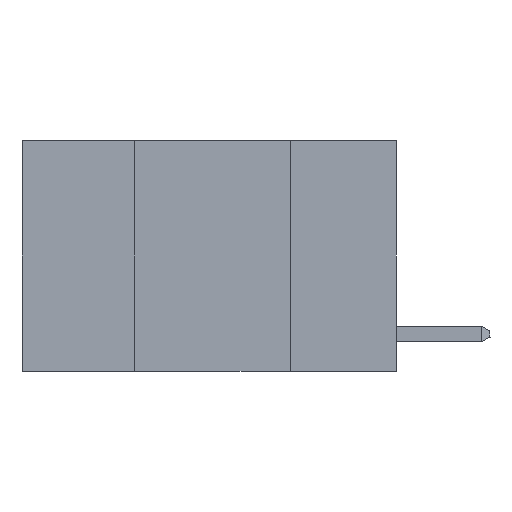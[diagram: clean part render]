
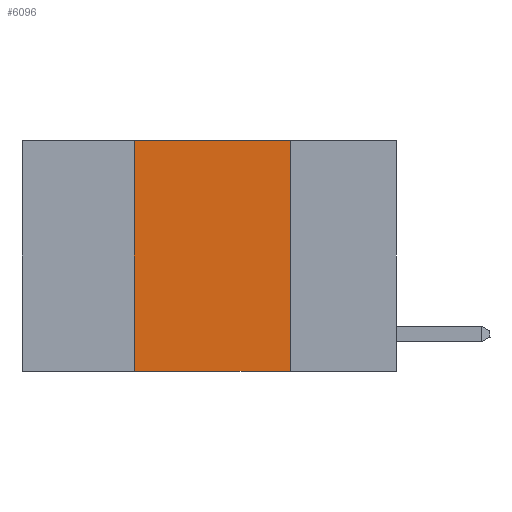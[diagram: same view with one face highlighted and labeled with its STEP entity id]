
A CAD part, left-side view. The second image highlights one B-rep face of the part: STEP entity #6096.
In plain terms, the highlighted planar face has unit normal (-1, 0, 0).
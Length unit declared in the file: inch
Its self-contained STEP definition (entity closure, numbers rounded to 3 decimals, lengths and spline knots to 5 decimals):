
#703 = VERTEX_POINT ( 'NONE', #11160 ) ;
#1280 = LINE ( 'NONE', #9103, #7799 ) ;
#1834 = EDGE_CURVE ( 'NONE', #3812, #3307, #11126, .T. ) ;
#1981 = VECTOR ( 'NONE', #5624, 39.37008 ) ;
#2698 = ORIENTED_EDGE ( 'NONE', *, *, #6928, .T. ) ;
#3307 = VERTEX_POINT ( 'NONE', #4515 ) ;
#3812 = VERTEX_POINT ( 'NONE', #14347 ) ;
#3843 = ORIENTED_EDGE ( 'NONE', *, *, #1834, .F. ) ;
#3962 = FACE_OUTER_BOUND ( 'NONE', #10571, .T. ) ;
#4505 = CARTESIAN_POINT ( 'NONE',  ( 0., 0.42, 0. ) ) ;
#4515 = CARTESIAN_POINT ( 'NONE',  ( 0., 0.17, 0. ) ) ;
#5047 = DIRECTION ( 'NONE',  ( 0., 0., -1. ) ) ;
#5151 = DIRECTION ( 'NONE',  ( 1., 0., 0. ) ) ;
#5517 = CARTESIAN_POINT ( 'NONE',  ( 0., 0.6, 0. ) ) ;
#5624 = DIRECTION ( 'NONE',  ( 0., 0., 1. ) ) ;
#6096 = ADVANCED_FACE ( 'NONE', ( #3962 ), #11874, .F. ) ;
#6123 = CARTESIAN_POINT ( 'NONE',  ( 0., 0.42, -0.37 ) ) ;
#6208 = CARTESIAN_POINT ( 'NONE',  ( 0., 0.6, 0. ) ) ;
#6257 = CARTESIAN_POINT ( 'NONE',  ( 0., 0.17, 0. ) ) ;
#6723 = DIRECTION ( 'NONE',  ( 0., -1., 0. ) ) ;
#6928 = EDGE_CURVE ( 'NONE', #13178, #703, #1280, .T. ) ;
#7799 = VECTOR ( 'NONE', #6723, 39.37008 ) ;
#8449 = VECTOR ( 'NONE', #5047, 39.37008 ) ;
#8719 = LINE ( 'NONE', #6257, #8449 ) ;
#9103 = CARTESIAN_POINT ( 'NONE',  ( 0., 0.6, -0.37 ) ) ;
#10084 = DIRECTION ( 'NONE',  ( 0., -1., 0. ) ) ;
#10571 = EDGE_LOOP ( 'NONE', ( #14606, #3843, #12795, #2698 ) ) ;
#11126 = LINE ( 'NONE', #5517, #13685 ) ;
#11160 = CARTESIAN_POINT ( 'NONE',  ( 0., 0.17, -0.37 ) ) ;
#11522 = EDGE_CURVE ( 'NONE', #13178, #3812, #13768, .T. ) ;
#11874 = PLANE ( 'NONE',  #13803 ) ;
#12795 = ORIENTED_EDGE ( 'NONE', *, *, #11522, .F. ) ;
#13178 = VERTEX_POINT ( 'NONE', #6123 ) ;
#13685 = VECTOR ( 'NONE', #10084, 39.37008 ) ;
#13768 = LINE ( 'NONE', #4505, #1981 ) ;
#13803 = AXIS2_PLACEMENT_3D ( 'NONE', #6208, #5151, #13913 ) ;
#13913 = DIRECTION ( 'NONE',  ( 0., 0., -1. ) ) ;
#14347 = CARTESIAN_POINT ( 'NONE',  ( 0., 0.42, 0. ) ) ;
#14602 = EDGE_CURVE ( 'NONE', #3307, #703, #8719, .T. ) ;
#14606 = ORIENTED_EDGE ( 'NONE', *, *, #14602, .F. ) ;
